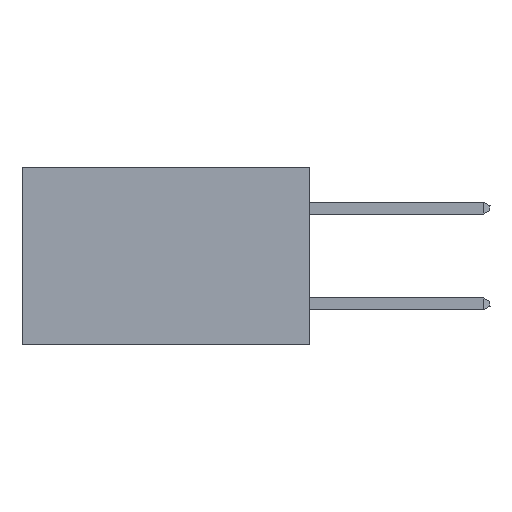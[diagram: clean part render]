
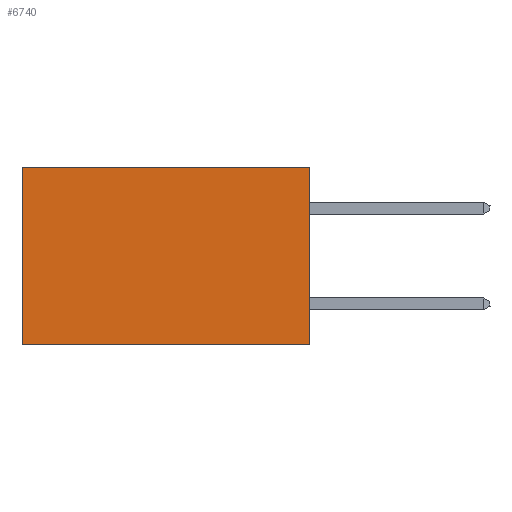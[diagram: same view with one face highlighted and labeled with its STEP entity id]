
A CAD part, left-side view. The second image highlights one B-rep face of the part: STEP entity #6740.
In plain terms, the highlighted planar face has unit normal (-1, 0, 0).
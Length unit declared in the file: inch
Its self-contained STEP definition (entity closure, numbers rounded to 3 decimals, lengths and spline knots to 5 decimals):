
#43 = VECTOR ( 'NONE', #1077, 39.37008 ) ;
#86 = LINE ( 'NONE', #3820, #8750 ) ;
#810 = EDGE_CURVE ( 'NONE', #5228, #6772, #2411, .T. ) ;
#951 = CARTESIAN_POINT ( 'NONE',  ( 0.2875, 0., 0. ) ) ;
#1072 = VERTEX_POINT ( 'NONE', #8039 ) ;
#1077 = DIRECTION ( 'NONE',  ( 0., 0., -1. ) ) ;
#1340 = LINE ( 'NONE', #8976, #7416 ) ;
#1561 = ORIENTED_EDGE ( 'NONE', *, *, #6468, .F. ) ;
#1835 = CARTESIAN_POINT ( 'NONE',  ( 0.2875, 0.6, -0.37 ) ) ;
#1841 = AXIS2_PLACEMENT_3D ( 'NONE', #8383, #6993, #7688 ) ;
#2188 = CARTESIAN_POINT ( 'NONE',  ( 0.2875, 0., -0.37 ) ) ;
#2411 = LINE ( 'NONE', #8373, #43 ) ;
#2535 = CARTESIAN_POINT ( 'NONE',  ( 0.2875, 0.6, 0. ) ) ;
#2777 = EDGE_CURVE ( 'NONE', #1072, #6213, #86, .T. ) ;
#3346 = ORIENTED_EDGE ( 'NONE', *, *, #2777, .F. ) ;
#3820 = CARTESIAN_POINT ( 'NONE',  ( 0.2875, 0., 0. ) ) ;
#4106 = EDGE_LOOP ( 'NONE', ( #6542, #1561, #3346, #6906 ) ) ;
#4638 = LINE ( 'NONE', #951, #7117 ) ;
#5228 = VERTEX_POINT ( 'NONE', #2535 ) ;
#5392 = EDGE_CURVE ( 'NONE', #1072, #5228, #4638, .T. ) ;
#6207 = PLANE ( 'NONE',  #1841 ) ;
#6213 = VERTEX_POINT ( 'NONE', #2188 ) ;
#6468 = EDGE_CURVE ( 'NONE', #6213, #6772, #1340, .T. ) ;
#6542 = ORIENTED_EDGE ( 'NONE', *, *, #810, .T. ) ;
#6740 = ADVANCED_FACE ( 'NONE', ( #8094 ), #6207, .F. ) ;
#6772 = VERTEX_POINT ( 'NONE', #1835 ) ;
#6906 = ORIENTED_EDGE ( 'NONE', *, *, #5392, .T. ) ;
#6993 = DIRECTION ( 'NONE',  ( 1., 0., 0. ) ) ;
#7117 = VECTOR ( 'NONE', #7290, 39.37008 ) ;
#7290 = DIRECTION ( 'NONE',  ( 0., 1., 0. ) ) ;
#7410 = DIRECTION ( 'NONE',  ( 0., 0., -1. ) ) ;
#7416 = VECTOR ( 'NONE', #8171, 39.37008 ) ;
#7688 = DIRECTION ( 'NONE',  ( 0., 0., -1. ) ) ;
#8039 = CARTESIAN_POINT ( 'NONE',  ( 0.2875, 0., 0. ) ) ;
#8094 = FACE_OUTER_BOUND ( 'NONE', #4106, .T. ) ;
#8171 = DIRECTION ( 'NONE',  ( 0., 1., 0. ) ) ;
#8373 = CARTESIAN_POINT ( 'NONE',  ( 0.2875, 0.6, 0. ) ) ;
#8383 = CARTESIAN_POINT ( 'NONE',  ( 0.2875, 0., 0. ) ) ;
#8750 = VECTOR ( 'NONE', #7410, 39.37008 ) ;
#8976 = CARTESIAN_POINT ( 'NONE',  ( 0.2875, 0., -0.37 ) ) ;
